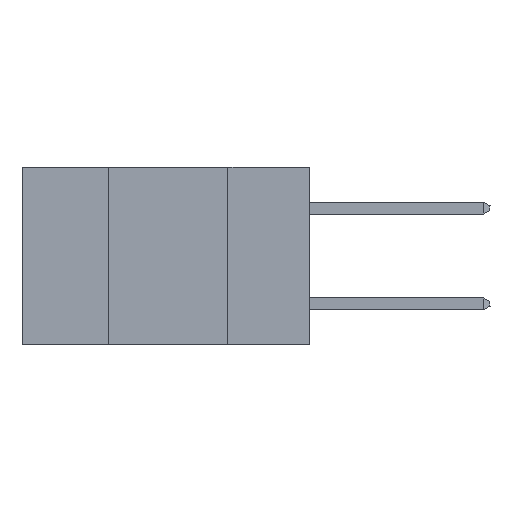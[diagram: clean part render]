
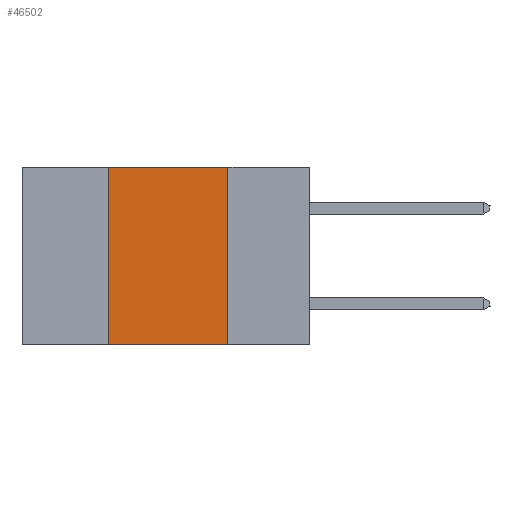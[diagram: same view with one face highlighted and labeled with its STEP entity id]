
A CAD part, left-side view. The second image highlights one B-rep face of the part: STEP entity #46502.
In plain terms, the highlighted planar face has unit normal (-1, 0, 0).
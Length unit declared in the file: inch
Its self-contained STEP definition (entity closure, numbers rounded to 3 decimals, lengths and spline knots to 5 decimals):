
#2298 = VERTEX_POINT ( 'NONE', #46152 ) ;
#2618 = DIRECTION ( 'NONE',  ( 1., 0., 0. ) ) ;
#3388 = CARTESIAN_POINT ( 'NONE',  ( 0., 0.6, 0. ) ) ;
#3862 = ORIENTED_EDGE ( 'NONE', *, *, #24155, .F. ) ;
#5002 = ORIENTED_EDGE ( 'NONE', *, *, #46369, .F. ) ;
#7383 = EDGE_LOOP ( 'NONE', ( #5002, #15339, #3862, #18741 ) ) ;
#7390 = DIRECTION ( 'NONE',  ( 0., -1., 0. ) ) ;
#8819 = VECTOR ( 'NONE', #44184, 39.37008 ) ;
#9523 = CARTESIAN_POINT ( 'NONE',  ( 0., 0.17, 0. ) ) ;
#9955 = LINE ( 'NONE', #9523, #21453 ) ;
#13037 = DIRECTION ( 'NONE',  ( 0., 0., -1. ) ) ;
#13957 = DIRECTION ( 'NONE',  ( 0., -1., 0. ) ) ;
#15339 = ORIENTED_EDGE ( 'NONE', *, *, #28835, .F. ) ;
#16805 = VECTOR ( 'NONE', #7390, 39.37008 ) ;
#17461 = CARTESIAN_POINT ( 'NONE',  ( 0., 0.6, -0.37 ) ) ;
#18594 = FACE_OUTER_BOUND ( 'NONE', #7383, .T. ) ;
#18741 = ORIENTED_EDGE ( 'NONE', *, *, #31285, .T. ) ;
#20867 = PLANE ( 'NONE',  #32476 ) ;
#21453 = VECTOR ( 'NONE', #35594, 39.37008 ) ;
#21635 = CARTESIAN_POINT ( 'NONE',  ( 0., 0.42, -0.37 ) ) ;
#23109 = VERTEX_POINT ( 'NONE', #42160 ) ;
#24155 = EDGE_CURVE ( 'NONE', #31537, #2298, #28300, .T. ) ;
#24581 = CARTESIAN_POINT ( 'NONE',  ( 0., 0.6, 0. ) ) ;
#28300 = LINE ( 'NONE', #33148, #8819 ) ;
#28835 = EDGE_CURVE ( 'NONE', #2298, #29890, #35124, .T. ) ;
#29890 = VERTEX_POINT ( 'NONE', #38494 ) ;
#30253 = VECTOR ( 'NONE', #13957, 39.37008 ) ;
#31285 = EDGE_CURVE ( 'NONE', #31537, #23109, #31995, .T. ) ;
#31537 = VERTEX_POINT ( 'NONE', #21635 ) ;
#31995 = LINE ( 'NONE', #17461, #30253 ) ;
#32476 = AXIS2_PLACEMENT_3D ( 'NONE', #24581, #2618, #13037 ) ;
#33148 = CARTESIAN_POINT ( 'NONE',  ( 0., 0.42, 0. ) ) ;
#35124 = LINE ( 'NONE', #3388, #16805 ) ;
#35594 = DIRECTION ( 'NONE',  ( 0., 0., -1. ) ) ;
#38494 = CARTESIAN_POINT ( 'NONE',  ( 0., 0.17, 0. ) ) ;
#42160 = CARTESIAN_POINT ( 'NONE',  ( 0., 0.17, -0.37 ) ) ;
#44184 = DIRECTION ( 'NONE',  ( 0., 0., 1. ) ) ;
#46152 = CARTESIAN_POINT ( 'NONE',  ( 0., 0.42, 0. ) ) ;
#46369 = EDGE_CURVE ( 'NONE', #29890, #23109, #9955, .T. ) ;
#46502 = ADVANCED_FACE ( 'NONE', ( #18594 ), #20867, .F. ) ;
